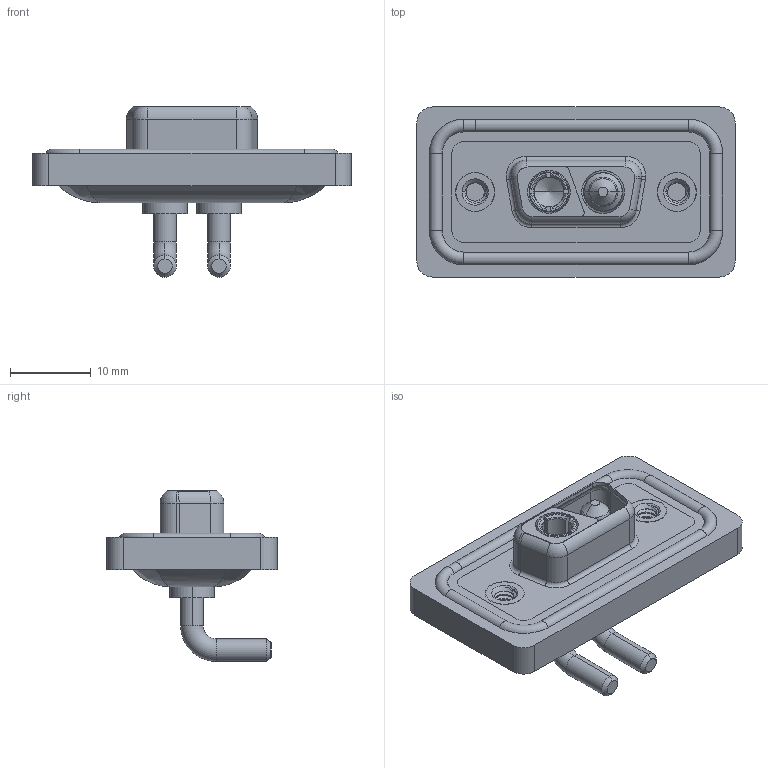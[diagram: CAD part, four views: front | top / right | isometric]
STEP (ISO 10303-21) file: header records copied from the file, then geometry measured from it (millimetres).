
FILE_DESCRIPTION (( 'STEP AP203' ), '1' );
FILE_NAME ('630W2WK2240-2N2.STEP', '2024-04-11T21:13:45', ( '' ), ( '' ), 'SwSTEP 2.0', 'SolidWorks 2023', '' );
FILE_SCHEMA (( 'CONFIG_CONTROL_DESIGN' ));
Length unit declared in the file: millimetre
Products named in the file (8): 630Combo Threaded Rivet_2; 630Combo Shell Front_09 Contacts; 630W2WK2240-2N2; 630Combo Shell Rear_09 Contacts; 630Combo Waterproof Housing_09 Contacts; 630Combo Housing_2WK2; Power Pin_20A RA; Power Socket_20A RA
Assembly tree (8 placements, depth 2):
  630W2WK2240-2N2
    630Combo Housing_2WK2
    630Combo Shell Front_09 Contacts
    630Combo Shell Rear_09 Contacts
    630Combo Threaded Rivet_2  x2
    Power Socket_20A RA
    Power Pin_20A RA
    630Combo Waterproof Housing_09 Contacts
Bounding box: 39.5 x 21.1 x 21.2 mm (x, y, z)
Volume: 4706.4 mm3; surface area: 7493.8 mm2
Topology: 11 solids, 11 shells, 508 faces, 1250 edges, 781 vertices
Faces by surface type: cylinder 235, plane 144, torus 81, cone 36, bspline 12
Entity records: 16848 total; most frequent: CARTESIAN_POINT 4641, DIRECTION 2506, ORIENTED_EDGE 2318, EDGE_CURVE 1159, AXIS2_PLACEMENT_3D 1007, VERTEX_POINT 729, CIRCLE 530, EDGE_LOOP 520
